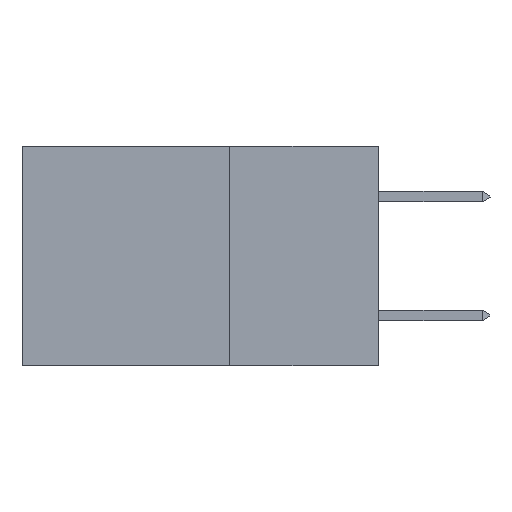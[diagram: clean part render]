
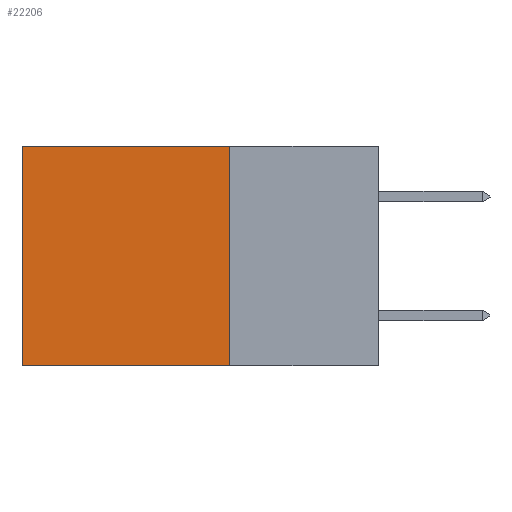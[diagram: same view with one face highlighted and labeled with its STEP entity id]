
A CAD part, left-side view. The second image highlights one B-rep face of the part: STEP entity #22206.
In plain terms, the highlighted planar face has unit normal (-1, 0, 0).
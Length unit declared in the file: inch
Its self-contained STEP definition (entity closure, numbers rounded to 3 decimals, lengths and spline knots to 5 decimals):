
#895 = VERTEX_POINT ( 'NONE', #17974 ) ;
#983 = DIRECTION ( 'NONE',  ( 0., 0., -1. ) ) ;
#1639 = ORIENTED_EDGE ( 'NONE', *, *, #24266, .F. ) ;
#2219 = EDGE_CURVE ( 'NONE', #16762, #895, #18777, .T. ) ;
#2471 = ORIENTED_EDGE ( 'NONE', *, *, #18867, .T. ) ;
#3051 = VECTOR ( 'NONE', #9702, 39.37008 ) ;
#3107 = LINE ( 'NONE', #20179, #22204 ) ;
#4355 = CARTESIAN_POINT ( 'NONE',  ( 0.298, 0.25, 0. ) ) ;
#8279 = ORIENTED_EDGE ( 'NONE', *, *, #9062, .T. ) ;
#9062 = EDGE_CURVE ( 'NONE', #13341, #23753, #19968, .T. ) ;
#9702 = DIRECTION ( 'NONE',  ( 0., 1., 0. ) ) ;
#10287 = CARTESIAN_POINT ( 'NONE',  ( 0.298, 0.6, 0. ) ) ;
#11241 = EDGE_LOOP ( 'NONE', ( #8279, #1639, #14129, #2471 ) ) ;
#12642 = CARTESIAN_POINT ( 'NONE',  ( 0.298, 0.25, 0. ) ) ;
#12948 = DIRECTION ( 'NONE',  ( 0., 0., -1. ) ) ;
#13341 = VERTEX_POINT ( 'NONE', #10287 ) ;
#14129 = ORIENTED_EDGE ( 'NONE', *, *, #2219, .F. ) ;
#14615 = CARTESIAN_POINT ( 'NONE',  ( 0.298, 0.6, 0. ) ) ;
#14674 = CARTESIAN_POINT ( 'NONE',  ( 0.298, 0.25, 0. ) ) ;
#14922 = DIRECTION ( 'NONE',  ( 1., 0., 0. ) ) ;
#16762 = VERTEX_POINT ( 'NONE', #4355 ) ;
#16921 = VECTOR ( 'NONE', #983, 39.37008 ) ;
#17020 = CARTESIAN_POINT ( 'NONE',  ( 0.298, 0.6, -0.37 ) ) ;
#17974 = CARTESIAN_POINT ( 'NONE',  ( 0.298, 0.25, -0.37 ) ) ;
#18526 = AXIS2_PLACEMENT_3D ( 'NONE', #14674, #14922, #12948 ) ;
#18777 = LINE ( 'NONE', #12642, #16921 ) ;
#18867 = EDGE_CURVE ( 'NONE', #16762, #13341, #3107, .T. ) ;
#19021 = DIRECTION ( 'NONE',  ( 0., 1., 0. ) ) ;
#19345 = CARTESIAN_POINT ( 'NONE',  ( 0.298, 0.25, -0.37 ) ) ;
#19968 = LINE ( 'NONE', #14615, #20276 ) ;
#20179 = CARTESIAN_POINT ( 'NONE',  ( 0.298, 0.25, 0. ) ) ;
#20276 = VECTOR ( 'NONE', #20346, 39.37008 ) ;
#20346 = DIRECTION ( 'NONE',  ( 0., 0., -1. ) ) ;
#22204 = VECTOR ( 'NONE', #19021, 39.37008 ) ;
#22206 = ADVANCED_FACE ( 'NONE', ( #22218 ), #22535, .F. ) ;
#22218 = FACE_OUTER_BOUND ( 'NONE', #11241, .T. ) ;
#22535 = PLANE ( 'NONE',  #18526 ) ;
#23753 = VERTEX_POINT ( 'NONE', #17020 ) ;
#24266 = EDGE_CURVE ( 'NONE', #895, #23753, #24929, .T. ) ;
#24929 = LINE ( 'NONE', #19345, #3051 ) ;
